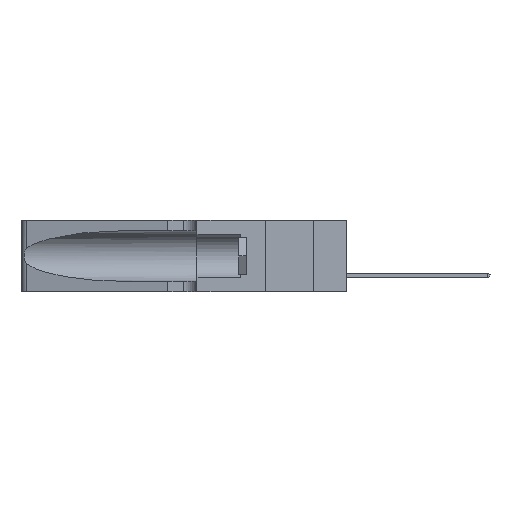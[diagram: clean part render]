
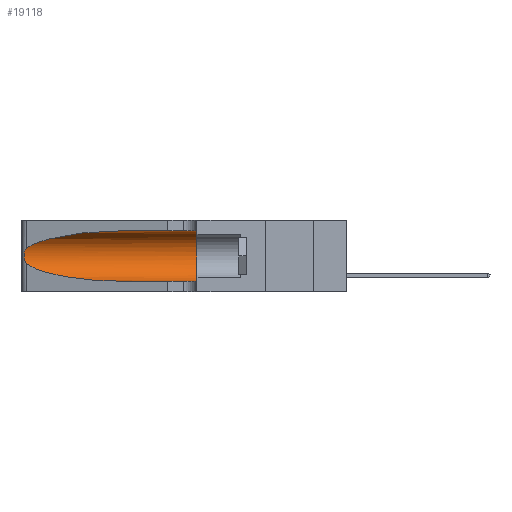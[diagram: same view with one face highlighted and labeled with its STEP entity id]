
A CAD part, left-side view. The second image highlights one B-rep face of the part: STEP entity #19118.
In plain terms, the highlighted cylindrical face has radius 3.308 mm (diameter 6.617 mm), a partial arc.
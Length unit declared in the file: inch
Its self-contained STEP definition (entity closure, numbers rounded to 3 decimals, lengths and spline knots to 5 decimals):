
#891 = AXIS2_PLACEMENT_3D ( 'NONE', #30772, #24344, #5374 ) ;
#2444 = FACE_OUTER_BOUND ( 'NONE', #30282, .T. ) ;
#2717 = CARTESIAN_POINT ( 'NONE',  ( 0.1305, 0.72297, 0.31525 ) ) ;
#2879 = CARTESIAN_POINT ( 'NONE',  ( 0.18966, 0.96281, 0.31525 ) ) ;
#3114 = CARTESIAN_POINT ( 'NONE',  ( 0.1305, 0.72297, 0.05475 ) ) ;
#3405 = CARTESIAN_POINT ( 'NONE',  ( 0.2373, 1.15595, 0.28018 ) ) ;
#4044 = B_SPLINE_CURVE_WITH_KNOTS ( 'NONE', 3,
 ( #4642, #4772, #16411, #19560, #37771, #25624, #9700, #34749, #16543, #8151, #22966, #7324, #13636, #30102 ),
 .UNSPECIFIED., .F., .F.,
 ( 4, 2, 2, 2, 2, 2, 4 ),
 ( 0., 0.00027, 0.00053, 0.00107, 0.0016, 0.00187, 0.00214 ),
 .UNSPECIFIED. ) ;
#4207 = CARTESIAN_POINT ( 'NONE',  ( 0.1305, 0.72297, 0.05475 ) ) ;
#4642 = CARTESIAN_POINT ( 'NONE',  ( 0.25487, 1.22718, 0.22369 ) ) ;
#4772 = CARTESIAN_POINT ( 'NONE',  ( 0.25555, 1.22994, 0.2215 ) ) ;
#5002 = CARTESIAN_POINT ( 'NONE',  ( 0.1305, 1.61858, 0.31525 ) ) ;
#5374 = DIRECTION ( 'NONE',  ( 0., 0., 1. ) ) ;
#5647 = EDGE_CURVE ( 'NONE', #8329, #26188, #31301, .T. ) ;
#5735 = ORIENTED_EDGE ( 'NONE', *, *, #10589, .T. ) ;
#5757 = ORIENTED_EDGE ( 'NONE', *, *, #23280, .F. ) ;
#6093 = CARTESIAN_POINT ( 'NONE',  ( 0.1305, 1.61858, 0.185 ) ) ;
#6464 = DIRECTION ( 'NONE',  ( 0., -1., 0. ) ) ;
#7132 = VECTOR ( 'NONE', #23261, 39.37008 ) ;
#7324 = CARTESIAN_POINT ( 'NONE',  ( 0.25639, 1.23186, 0.15144 ) ) ;
#8151 = CARTESIAN_POINT ( 'NONE',  ( 0.25856, 1.23593, 0.16098 ) ) ;
#8329 = VERTEX_POINT ( 'NONE', #2717 ) ;
#9700 = CARTESIAN_POINT ( 'NONE',  ( 0.26075, 1.23896, 0.19203 ) ) ;
#10589 = EDGE_CURVE ( 'NONE', #30782, #13539, #21880, .T. ) ;
#11089 = AXIS2_PLACEMENT_3D ( 'NONE', #6093, #6464, #17706 ) ;
#11276 = ORIENTED_EDGE ( 'NONE', *, *, #5647, .F. ) ;
#11349 = CYLINDRICAL_SURFACE ( 'NONE', #11089, 0.13025 ) ;
#12118 =( BOUNDED_CURVE ( )  B_SPLINE_CURVE ( 3, ( #12234, #2879, #3405, #37982 ),
 .UNSPECIFIED., .F., .F. ) 
 B_SPLINE_CURVE_WITH_KNOTS ( ( 4, 4 ),
 ( 1.5708, 2.84003 ),
 .UNSPECIFIED. ) 
 CURVE ( )  GEOMETRIC_REPRESENTATION_ITEM ( )  RATIONAL_B_SPLINE_CURVE ( ( 1., 0.87, 0.87, 1. ) ) 
 REPRESENTATION_ITEM ( '' )  );
#12234 = CARTESIAN_POINT ( 'NONE',  ( 0.1305, 0.72297, 0.31525 ) ) ;
#13539 = VERTEX_POINT ( 'NONE', #29712 ) ;
#13636 = CARTESIAN_POINT ( 'NONE',  ( 0.25555, 1.22993, 0.14849 ) ) ;
#13777 = VERTEX_POINT ( 'NONE', #40211 ) ;
#15018 = CIRCLE ( 'NONE', #891, 0.13025 ) ;
#16411 = CARTESIAN_POINT ( 'NONE',  ( 0.25639, 1.23184, 0.21858 ) ) ;
#16543 = CARTESIAN_POINT ( 'NONE',  ( 0.26017, 1.23833, 0.17102 ) ) ;
#17244 = CARTESIAN_POINT ( 'NONE',  ( 0.1305, 1.61858, 0.05475 ) ) ;
#17253 = ORIENTED_EDGE ( 'NONE', *, *, #32304, .T. ) ;
#17706 = DIRECTION ( 'NONE',  ( 0., 0., -1. ) ) ;
#18819 = CARTESIAN_POINT ( 'NONE',  ( 0.25487, 1.22718, 0.14631 ) ) ;
#19118 = ADVANCED_FACE ( 'NONE', ( #2444 ), #11349, .F. ) ;
#19560 = CARTESIAN_POINT ( 'NONE',  ( 0.25787, 1.23484, 0.2124 ) ) ;
#20560 = DIRECTION ( 'NONE',  ( 0., -1., 0. ) ) ;
#21880 = LINE ( 'NONE', #17244, #7132 ) ;
#21946 = CARTESIAN_POINT ( 'NONE',  ( 0.18966, 0.96281, 0.05475 ) ) ;
#22439 =( BOUNDED_CURVE ( )  B_SPLINE_CURVE ( 3, ( #18819, #40738, #21946, #3114 ),
 .UNSPECIFIED., .F., .F. ) 
 B_SPLINE_CURVE_WITH_KNOTS ( ( 4, 4 ),
 ( 3.44316, 4.71239 ),
 .UNSPECIFIED. ) 
 CURVE ( )  GEOMETRIC_REPRESENTATION_ITEM ( )  RATIONAL_B_SPLINE_CURVE ( ( 1., 0.87, 0.87, 1. ) ) 
 REPRESENTATION_ITEM ( '' )  );
#22536 = EDGE_CURVE ( 'NONE', #32801, #13777, #4044, .T. ) ;
#22966 = CARTESIAN_POINT ( 'NONE',  ( 0.25789, 1.23486, 0.15765 ) ) ;
#23261 = DIRECTION ( 'NONE',  ( 0., -1., 0. ) ) ;
#23280 = EDGE_CURVE ( 'NONE', #26188, #13539, #15018, .T. ) ;
#24344 = DIRECTION ( 'NONE',  ( 0., 1., 0. ) ) ;
#24426 = CARTESIAN_POINT ( 'NONE',  ( 0.25487, 1.22718, 0.22369 ) ) ;
#25624 = CARTESIAN_POINT ( 'NONE',  ( 0.26018, 1.23835, 0.19895 ) ) ;
#26188 = VERTEX_POINT ( 'NONE', #26574 ) ;
#26574 = CARTESIAN_POINT ( 'NONE',  ( 0.1305, 0.35, 0.31525 ) ) ;
#27924 = EDGE_CURVE ( 'NONE', #13777, #30782, #22439, .T. ) ;
#29712 = CARTESIAN_POINT ( 'NONE',  ( 0.1305, 0.35, 0.05475 ) ) ;
#30102 = CARTESIAN_POINT ( 'NONE',  ( 0.25487, 1.22718, 0.14631 ) ) ;
#30282 = EDGE_LOOP ( 'NONE', ( #17253, #34586, #40630, #5735, #5757, #11276 ) ) ;
#30772 = CARTESIAN_POINT ( 'NONE',  ( 0.1305, 0.35, 0.185 ) ) ;
#30782 = VERTEX_POINT ( 'NONE', #4207 ) ;
#31301 = LINE ( 'NONE', #5002, #32239 ) ;
#32239 = VECTOR ( 'NONE', #20560, 39.37008 ) ;
#32304 = EDGE_CURVE ( 'NONE', #8329, #32801, #12118, .T. ) ;
#32801 = VERTEX_POINT ( 'NONE', #24426 ) ;
#34586 = ORIENTED_EDGE ( 'NONE', *, *, #22536, .T. ) ;
#34749 = CARTESIAN_POINT ( 'NONE',  ( 0.26075, 1.23896, 0.178 ) ) ;
#37771 = CARTESIAN_POINT ( 'NONE',  ( 0.25854, 1.2359, 0.20912 ) ) ;
#37982 = CARTESIAN_POINT ( 'NONE',  ( 0.25487, 1.22718, 0.22369 ) ) ;
#40211 = CARTESIAN_POINT ( 'NONE',  ( 0.25487, 1.22718, 0.14631 ) ) ;
#40630 = ORIENTED_EDGE ( 'NONE', *, *, #27924, .T. ) ;
#40738 = CARTESIAN_POINT ( 'NONE',  ( 0.2373, 1.15595, 0.08982 ) ) ;
